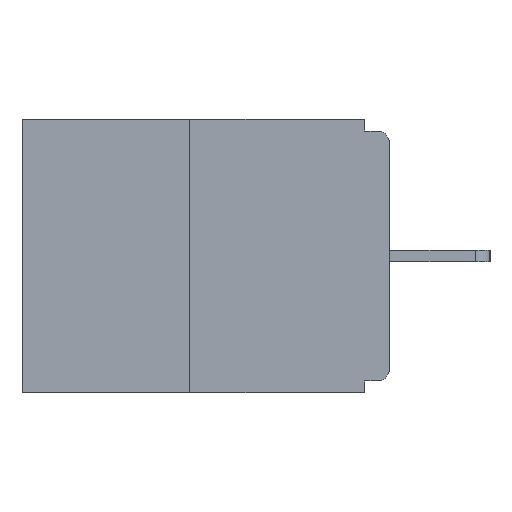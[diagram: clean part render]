
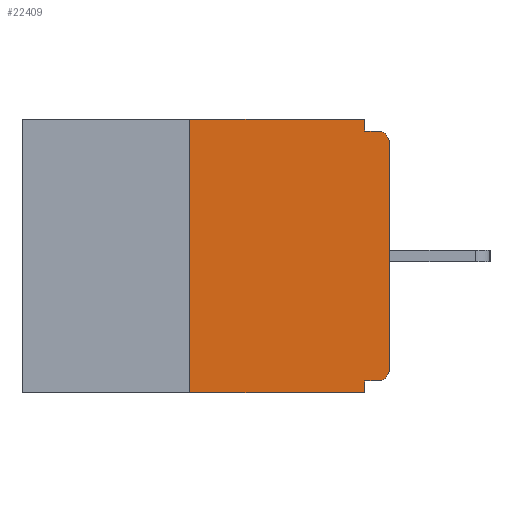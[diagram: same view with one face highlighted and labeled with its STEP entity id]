
A CAD part, left-side view. The second image highlights one B-rep face of the part: STEP entity #22409.
In plain terms, the highlighted planar face has unit normal (-1, 0, 0).
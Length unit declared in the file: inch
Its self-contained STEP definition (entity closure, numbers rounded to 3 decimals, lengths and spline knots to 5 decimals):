
#230 = ORIENTED_EDGE ( 'NONE', *, *, #2989, .F. ) ;
#535 = VECTOR ( 'NONE', #16568, 39.37008 ) ;
#957 = EDGE_CURVE ( 'NONE', #21265, #14611, #21681, .T. ) ;
#1389 = ORIENTED_EDGE ( 'NONE', *, *, #16148, .F. ) ;
#1736 = DIRECTION ( 'NONE',  ( 0., -1., 0. ) ) ;
#1771 = DIRECTION ( 'NONE',  ( 0., 0., -1. ) ) ;
#1873 = LINE ( 'NONE', #20516, #10149 ) ;
#2016 = CARTESIAN_POINT ( 'NONE',  ( 0., 0.46, 0. ) ) ;
#2049 = CARTESIAN_POINT ( 'NONE',  ( 0., 0.25, 0. ) ) ;
#2069 = VERTEX_POINT ( 'NONE', #12600 ) ;
#2433 = VERTEX_POINT ( 'NONE', #14060 ) ;
#2464 = CIRCLE ( 'NONE', #10643, 0.015 ) ;
#2989 = EDGE_CURVE ( 'NONE', #14611, #2433, #18086, .T. ) ;
#3039 = CARTESIAN_POINT ( 'NONE',  ( 0., 0., -0.328 ) ) ;
#3962 = CARTESIAN_POINT ( 'NONE',  ( 0., 0.015, -0.328 ) ) ;
#4092 = VERTEX_POINT ( 'NONE', #17407 ) ;
#4141 = CARTESIAN_POINT ( 'NONE',  ( 0., 0.46, 0. ) ) ;
#4186 = DIRECTION ( 'NONE',  ( 0., -1., 0. ) ) ;
#5105 = ORIENTED_EDGE ( 'NONE', *, *, #22966, .F. ) ;
#6102 = CIRCLE ( 'NONE', #19800, 0.015 ) ;
#6221 = LINE ( 'NONE', #4141, #7653 ) ;
#6239 = DIRECTION ( 'NONE',  ( -1., 0., 0. ) ) ;
#6272 = DIRECTION ( 'NONE',  ( 0., 0., 1. ) ) ;
#6306 = VERTEX_POINT ( 'NONE', #2049 ) ;
#6597 = DIRECTION ( 'NONE',  ( 0., 0., 1. ) ) ;
#7080 = VECTOR ( 'NONE', #7140, 39.37008 ) ;
#7140 = DIRECTION ( 'NONE',  ( 0., -1., 0. ) ) ;
#7284 = PLANE ( 'NONE',  #20571 ) ;
#7409 = DIRECTION ( 'NONE',  ( -1., 0., 0. ) ) ;
#7653 = VECTOR ( 'NONE', #1736, 39.37008 ) ;
#7871 = ORIENTED_EDGE ( 'NONE', *, *, #19548, .F. ) ;
#7907 = CARTESIAN_POINT ( 'NONE',  ( 0., 0.25, -0.343 ) ) ;
#8006 = EDGE_CURVE ( 'NONE', #2069, #17576, #13995, .T. ) ;
#8665 = VECTOR ( 'NONE', #23731, 39.37008 ) ;
#9490 = DIRECTION ( 'NONE',  ( 1., 0., 0. ) ) ;
#9933 = VERTEX_POINT ( 'NONE', #12021 ) ;
#10149 = VECTOR ( 'NONE', #4186, 39.37008 ) ;
#10252 = VECTOR ( 'NONE', #12596, 39.37008 ) ;
#10643 = AXIS2_PLACEMENT_3D ( 'NONE', #17398, #6239, #11979 ) ;
#11018 = ORIENTED_EDGE ( 'NONE', *, *, #23661, .T. ) ;
#11081 = FACE_OUTER_BOUND ( 'NONE', #19521, .T. ) ;
#11155 = CARTESIAN_POINT ( 'NONE',  ( 0., 0.031, -0.328 ) ) ;
#11979 = DIRECTION ( 'NONE',  ( 0., 0., -1. ) ) ;
#12021 = CARTESIAN_POINT ( 'NONE',  ( 0., 0.031, 0. ) ) ;
#12197 = VECTOR ( 'NONE', #6272, 39.37008 ) ;
#12402 = LINE ( 'NONE', #14363, #7080 ) ;
#12596 = DIRECTION ( 'NONE',  ( 0., 1., 0. ) ) ;
#12600 = CARTESIAN_POINT ( 'NONE',  ( 0., 0., -0.313 ) ) ;
#13995 = LINE ( 'NONE', #23086, #12197 ) ;
#14060 = CARTESIAN_POINT ( 'NONE',  ( 0., 0.031, -0.343 ) ) ;
#14273 = EDGE_CURVE ( 'NONE', #17046, #2433, #1873, .T. ) ;
#14363 = CARTESIAN_POINT ( 'NONE',  ( 0., 0., -0.015 ) ) ;
#14385 = CARTESIAN_POINT ( 'NONE',  ( 0., 0.015, -0.313 ) ) ;
#14611 = VERTEX_POINT ( 'NONE', #11155 ) ;
#15586 = ORIENTED_EDGE ( 'NONE', *, *, #18215, .F. ) ;
#16148 = EDGE_CURVE ( 'NONE', #4092, #20014, #12402, .T. ) ;
#16255 = CARTESIAN_POINT ( 'NONE',  ( 0., 0.031, -0.343 ) ) ;
#16568 = DIRECTION ( 'NONE',  ( 0., 0., -1. ) ) ;
#16726 = DIRECTION ( 'NONE',  ( 0., 0., -1. ) ) ;
#17046 = VERTEX_POINT ( 'NONE', #7907 ) ;
#17398 = CARTESIAN_POINT ( 'NONE',  ( 0., 0.015, -0.03 ) ) ;
#17407 = CARTESIAN_POINT ( 'NONE',  ( 0., 0.031, -0.015 ) ) ;
#17576 = VERTEX_POINT ( 'NONE', #22474 ) ;
#17983 = CARTESIAN_POINT ( 'NONE',  ( 0., 0.25, 0. ) ) ;
#18074 = EDGE_CURVE ( 'NONE', #17576, #20014, #2464, .T. ) ;
#18086 = LINE ( 'NONE', #16255, #8665 ) ;
#18150 = LINE ( 'NONE', #18525, #535 ) ;
#18215 = EDGE_CURVE ( 'NONE', #17046, #6306, #23749, .T. ) ;
#18525 = CARTESIAN_POINT ( 'NONE',  ( 0., 0.031, 0. ) ) ;
#18971 = ORIENTED_EDGE ( 'NONE', *, *, #18074, .T. ) ;
#19521 = EDGE_LOOP ( 'NONE', ( #5105, #15586, #21474, #230, #20955, #11018, #23948, #18971, #1389, #7871 ) ) ;
#19548 = EDGE_CURVE ( 'NONE', #9933, #4092, #18150, .T. ) ;
#19726 = CARTESIAN_POINT ( 'NONE',  ( 0., 0.015, -0.015 ) ) ;
#19800 = AXIS2_PLACEMENT_3D ( 'NONE', #14385, #7409, #16726 ) ;
#20014 = VERTEX_POINT ( 'NONE', #19726 ) ;
#20516 = CARTESIAN_POINT ( 'NONE',  ( 0., 0.46, -0.343 ) ) ;
#20571 = AXIS2_PLACEMENT_3D ( 'NONE', #2016, #9490, #1771 ) ;
#20955 = ORIENTED_EDGE ( 'NONE', *, *, #957, .F. ) ;
#21265 = VERTEX_POINT ( 'NONE', #3962 ) ;
#21474 = ORIENTED_EDGE ( 'NONE', *, *, #14273, .T. ) ;
#21681 = LINE ( 'NONE', #3039, #10252 ) ;
#22008 = VECTOR ( 'NONE', #6597, 39.37008 ) ;
#22409 = ADVANCED_FACE ( 'NONE', ( #11081 ), #7284, .F. ) ;
#22474 = CARTESIAN_POINT ( 'NONE',  ( 0., 0., -0.03 ) ) ;
#22966 = EDGE_CURVE ( 'NONE', #6306, #9933, #6221, .T. ) ;
#23086 = CARTESIAN_POINT ( 'NONE',  ( 0., 0., 0. ) ) ;
#23661 = EDGE_CURVE ( 'NONE', #21265, #2069, #6102, .T. ) ;
#23731 = DIRECTION ( 'NONE',  ( 0., 0., -1. ) ) ;
#23749 = LINE ( 'NONE', #17983, #22008 ) ;
#23948 = ORIENTED_EDGE ( 'NONE', *, *, #8006, .T. ) ;
